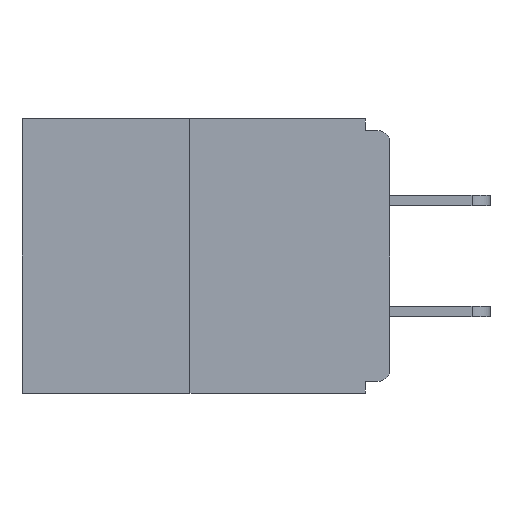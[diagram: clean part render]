
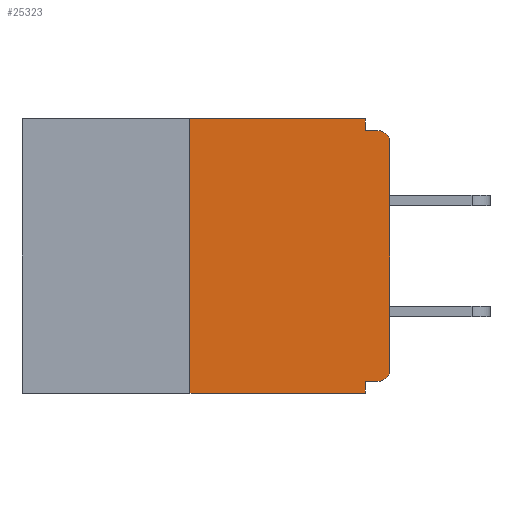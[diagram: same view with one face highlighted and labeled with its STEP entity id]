
A CAD part, left-side view. The second image highlights one B-rep face of the part: STEP entity #25323.
In plain terms, the highlighted planar face has unit normal (-1, 0, 0).
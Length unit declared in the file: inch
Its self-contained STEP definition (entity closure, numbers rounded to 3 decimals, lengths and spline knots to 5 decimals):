
#4 = DIRECTION ( 'NONE',  ( 0., 0., -1. ) ) ;
#327 = LINE ( 'NONE', #17256, #11149 ) ;
#756 = DIRECTION ( 'NONE',  ( 0., -1., 0. ) ) ;
#909 = VERTEX_POINT ( 'NONE', #15070 ) ;
#1015 = LINE ( 'NONE', #25570, #5338 ) ;
#1706 = EDGE_CURVE ( 'NONE', #909, #13571, #327, .T. ) ;
#2066 = VECTOR ( 'NONE', #4745, 39.37008 ) ;
#3191 = AXIS2_PLACEMENT_3D ( 'NONE', #23333, #3828, #13595 ) ;
#3629 = VERTEX_POINT ( 'NONE', #12218 ) ;
#3800 = LINE ( 'NONE', #20703, #24187 ) ;
#3828 = DIRECTION ( 'NONE',  ( 1., 0., 0. ) ) ;
#4385 = EDGE_CURVE ( 'NONE', #19233, #10772, #5067, .T. ) ;
#4745 = DIRECTION ( 'NONE',  ( 0., 0., 1. ) ) ;
#4758 = CARTESIAN_POINT ( 'NONE',  ( 0., 0.015, -0.313 ) ) ;
#5067 = CIRCLE ( 'NONE', #10935, 0.015 ) ;
#5165 = DIRECTION ( 'NONE',  ( 0., -1., 0. ) ) ;
#5338 = VECTOR ( 'NONE', #4, 39.37008 ) ;
#5510 = DIRECTION ( 'NONE',  ( 0., 0., -1. ) ) ;
#6274 = VECTOR ( 'NONE', #5165, 39.37008 ) ;
#6387 = ORIENTED_EDGE ( 'NONE', *, *, #11939, .T. ) ;
#7356 = EDGE_LOOP ( 'NONE', ( #18342, #16420, #6387, #13395, #14447, #21211, #12318, #9464, #24111, #11109 ) ) ;
#7376 = DIRECTION ( 'NONE',  ( 0., 0., 1. ) ) ;
#7538 = VECTOR ( 'NONE', #756, 39.37008 ) ;
#8497 = CIRCLE ( 'NONE', #15719, 0.015 ) ;
#9046 = CARTESIAN_POINT ( 'NONE',  ( 0., 0., -0.328 ) ) ;
#9362 = CARTESIAN_POINT ( 'NONE',  ( 0., 0., -0.313 ) ) ;
#9408 = EDGE_CURVE ( 'NONE', #3629, #12366, #8497, .T. ) ;
#9436 = CARTESIAN_POINT ( 'NONE',  ( 0., 0., 0. ) ) ;
#9464 = ORIENTED_EDGE ( 'NONE', *, *, #9408, .T. ) ;
#9922 = CARTESIAN_POINT ( 'NONE',  ( 0., 0.25, 0. ) ) ;
#9956 = CARTESIAN_POINT ( 'NONE',  ( 0., 0.031, 0. ) ) ;
#10352 = CARTESIAN_POINT ( 'NONE',  ( 0., 0.015, -0.015 ) ) ;
#10480 = EDGE_CURVE ( 'NONE', #11063, #21300, #12780, .T. ) ;
#10593 = CARTESIAN_POINT ( 'NONE',  ( 0., 0., -0.015 ) ) ;
#10649 = CARTESIAN_POINT ( 'NONE',  ( 0., 0.25, 0. ) ) ;
#10772 = VERTEX_POINT ( 'NONE', #9362 ) ;
#10806 = DIRECTION ( 'NONE',  ( 0., 1., 0. ) ) ;
#10935 = AXIS2_PLACEMENT_3D ( 'NONE', #4758, #20529, #18452 ) ;
#10971 = EDGE_CURVE ( 'NONE', #21300, #18722, #1015, .T. ) ;
#11022 = CARTESIAN_POINT ( 'NONE',  ( 0., 0.031, -0.343 ) ) ;
#11063 = VERTEX_POINT ( 'NONE', #9922 ) ;
#11109 = ORIENTED_EDGE ( 'NONE', *, *, #10971, .F. ) ;
#11149 = VECTOR ( 'NONE', #25519, 39.37008 ) ;
#11865 = LINE ( 'NONE', #10593, #7538 ) ;
#11939 = EDGE_CURVE ( 'NONE', #18432, #13571, #3800, .T. ) ;
#12057 = LINE ( 'NONE', #9436, #16414 ) ;
#12218 = CARTESIAN_POINT ( 'NONE',  ( 0., 0., -0.03 ) ) ;
#12318 = ORIENTED_EDGE ( 'NONE', *, *, #17497, .T. ) ;
#12366 = VERTEX_POINT ( 'NONE', #10352 ) ;
#12780 = LINE ( 'NONE', #12956, #6274 ) ;
#12956 = CARTESIAN_POINT ( 'NONE',  ( 0., 0.46, 0. ) ) ;
#13031 = EDGE_CURVE ( 'NONE', #19233, #909, #13938, .T. ) ;
#13395 = ORIENTED_EDGE ( 'NONE', *, *, #1706, .F. ) ;
#13571 = VERTEX_POINT ( 'NONE', #11022 ) ;
#13595 = DIRECTION ( 'NONE',  ( 0., 0., -1. ) ) ;
#13938 = LINE ( 'NONE', #9046, #23194 ) ;
#14447 = ORIENTED_EDGE ( 'NONE', *, *, #13031, .F. ) ;
#15070 = CARTESIAN_POINT ( 'NONE',  ( 0., 0.031, -0.328 ) ) ;
#15359 = PLANE ( 'NONE',  #3191 ) ;
#15719 = AXIS2_PLACEMENT_3D ( 'NONE', #19181, #25116, #5510 ) ;
#16414 = VECTOR ( 'NONE', #7376, 39.37008 ) ;
#16420 = ORIENTED_EDGE ( 'NONE', *, *, #19551, .F. ) ;
#17256 = CARTESIAN_POINT ( 'NONE',  ( 0., 0.031, -0.343 ) ) ;
#17497 = EDGE_CURVE ( 'NONE', #10772, #3629, #12057, .T. ) ;
#18342 = ORIENTED_EDGE ( 'NONE', *, *, #10480, .F. ) ;
#18432 = VERTEX_POINT ( 'NONE', #20789 ) ;
#18452 = DIRECTION ( 'NONE',  ( 0., 0., -1. ) ) ;
#18722 = VERTEX_POINT ( 'NONE', #20891 ) ;
#19181 = CARTESIAN_POINT ( 'NONE',  ( 0., 0.015, -0.03 ) ) ;
#19233 = VERTEX_POINT ( 'NONE', #19311 ) ;
#19311 = CARTESIAN_POINT ( 'NONE',  ( 0., 0.015, -0.328 ) ) ;
#19551 = EDGE_CURVE ( 'NONE', #18432, #11063, #19695, .T. ) ;
#19695 = LINE ( 'NONE', #10649, #2066 ) ;
#20529 = DIRECTION ( 'NONE',  ( -1., 0., 0. ) ) ;
#20703 = CARTESIAN_POINT ( 'NONE',  ( 0., 0.46, -0.343 ) ) ;
#20789 = CARTESIAN_POINT ( 'NONE',  ( 0., 0.25, -0.343 ) ) ;
#20891 = CARTESIAN_POINT ( 'NONE',  ( 0., 0.031, -0.015 ) ) ;
#20932 = DIRECTION ( 'NONE',  ( 0., -1., 0. ) ) ;
#21211 = ORIENTED_EDGE ( 'NONE', *, *, #4385, .T. ) ;
#21300 = VERTEX_POINT ( 'NONE', #9956 ) ;
#23194 = VECTOR ( 'NONE', #10806, 39.37008 ) ;
#23333 = CARTESIAN_POINT ( 'NONE',  ( 0., 0.46, 0. ) ) ;
#24111 = ORIENTED_EDGE ( 'NONE', *, *, #24655, .F. ) ;
#24186 = FACE_OUTER_BOUND ( 'NONE', #7356, .T. ) ;
#24187 = VECTOR ( 'NONE', #20932, 39.37008 ) ;
#24655 = EDGE_CURVE ( 'NONE', #18722, #12366, #11865, .T. ) ;
#25116 = DIRECTION ( 'NONE',  ( -1., 0., 0. ) ) ;
#25323 = ADVANCED_FACE ( 'NONE', ( #24186 ), #15359, .F. ) ;
#25519 = DIRECTION ( 'NONE',  ( 0., 0., -1. ) ) ;
#25570 = CARTESIAN_POINT ( 'NONE',  ( 0., 0.031, 0. ) ) ;
